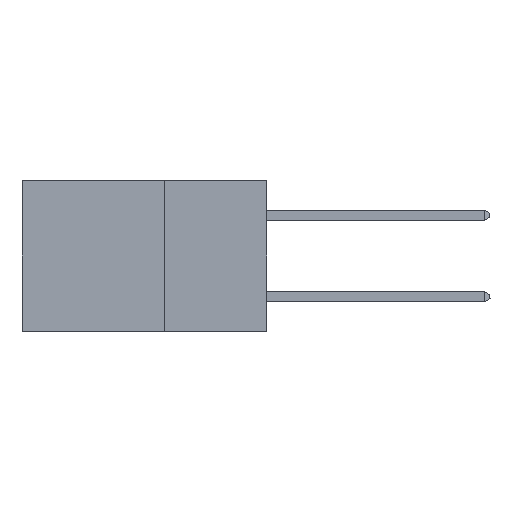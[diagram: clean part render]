
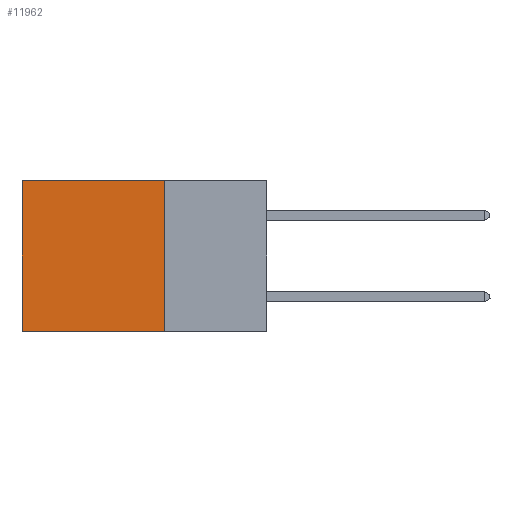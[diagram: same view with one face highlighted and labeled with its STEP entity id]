
A CAD part, left-side view. The second image highlights one B-rep face of the part: STEP entity #11962.
In plain terms, the highlighted planar face has unit normal (-1, 0, 0).
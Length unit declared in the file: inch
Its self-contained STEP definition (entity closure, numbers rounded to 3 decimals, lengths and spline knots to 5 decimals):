
#17 = AXIS2_PLACEMENT_3D ( 'NONE', #2624, #2820, #12585 ) ;
#39 = CARTESIAN_POINT ( 'NONE',  ( 0.2875, 0.6, 0. ) ) ;
#763 = PLANE ( 'NONE',  #17 ) ;
#1140 = EDGE_CURVE ( 'NONE', #12052, #5509, #2945, .T. ) ;
#2040 = CARTESIAN_POINT ( 'NONE',  ( 0.2875, 0.25, 0. ) ) ;
#2624 = CARTESIAN_POINT ( 'NONE',  ( 0.2875, 0.25, 0. ) ) ;
#2820 = DIRECTION ( 'NONE',  ( 1., 0., 0. ) ) ;
#2865 = CARTESIAN_POINT ( 'NONE',  ( 0.2875, 0.25, 0. ) ) ;
#2945 = LINE ( 'NONE', #9908, #4537 ) ;
#3655 = VERTEX_POINT ( 'NONE', #10559 ) ;
#3910 = ORIENTED_EDGE ( 'NONE', *, *, #10721, .F. ) ;
#4095 = VECTOR ( 'NONE', #9819, 39.37008 ) ;
#4537 = VECTOR ( 'NONE', #10985, 39.37008 ) ;
#5166 = ORIENTED_EDGE ( 'NONE', *, *, #5800, .F. ) ;
#5509 = VERTEX_POINT ( 'NONE', #39 ) ;
#5800 = EDGE_CURVE ( 'NONE', #10627, #3655, #11205, .T. ) ;
#5916 = LINE ( 'NONE', #2865, #4095 ) ;
#6745 = EDGE_CURVE ( 'NONE', #5509, #3655, #12568, .T. ) ;
#7353 = CARTESIAN_POINT ( 'NONE',  ( 0.2875, 0.25, -0.37 ) ) ;
#7450 = CARTESIAN_POINT ( 'NONE',  ( 0.2875, 0.25, -0.37 ) ) ;
#7636 = CARTESIAN_POINT ( 'NONE',  ( 0.2875, 0.6, 0. ) ) ;
#7840 = VECTOR ( 'NONE', #9224, 39.37008 ) ;
#9224 = DIRECTION ( 'NONE',  ( 0., 1., 0. ) ) ;
#9819 = DIRECTION ( 'NONE',  ( 0., 0., -1. ) ) ;
#9908 = CARTESIAN_POINT ( 'NONE',  ( 0.2875, 0.25, 0. ) ) ;
#10559 = CARTESIAN_POINT ( 'NONE',  ( 0.2875, 0.6, -0.37 ) ) ;
#10627 = VERTEX_POINT ( 'NONE', #7450 ) ;
#10721 = EDGE_CURVE ( 'NONE', #12052, #10627, #5916, .T. ) ;
#10985 = DIRECTION ( 'NONE',  ( 0., 1., 0. ) ) ;
#11205 = LINE ( 'NONE', #7353, #7840 ) ;
#11375 = FACE_OUTER_BOUND ( 'NONE', #12580, .T. ) ;
#11484 = DIRECTION ( 'NONE',  ( 0., 0., -1. ) ) ;
#11953 = VECTOR ( 'NONE', #11484, 39.37008 ) ;
#11962 = ADVANCED_FACE ( 'NONE', ( #11375 ), #763, .F. ) ;
#12052 = VERTEX_POINT ( 'NONE', #2040 ) ;
#12170 = ORIENTED_EDGE ( 'NONE', *, *, #6745, .T. ) ;
#12173 = ORIENTED_EDGE ( 'NONE', *, *, #1140, .T. ) ;
#12568 = LINE ( 'NONE', #7636, #11953 ) ;
#12580 = EDGE_LOOP ( 'NONE', ( #12170, #5166, #3910, #12173 ) ) ;
#12585 = DIRECTION ( 'NONE',  ( 0., 0., -1. ) ) ;
